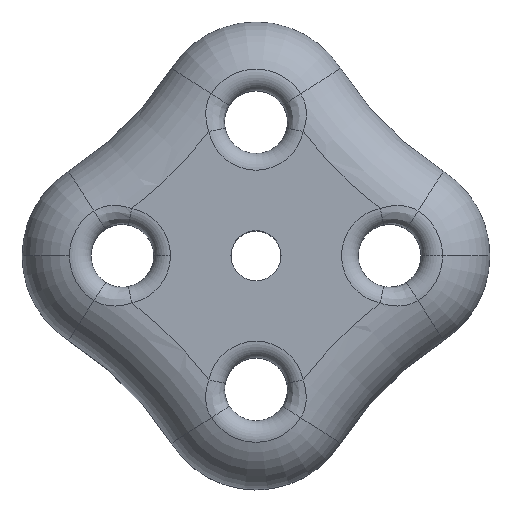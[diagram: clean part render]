
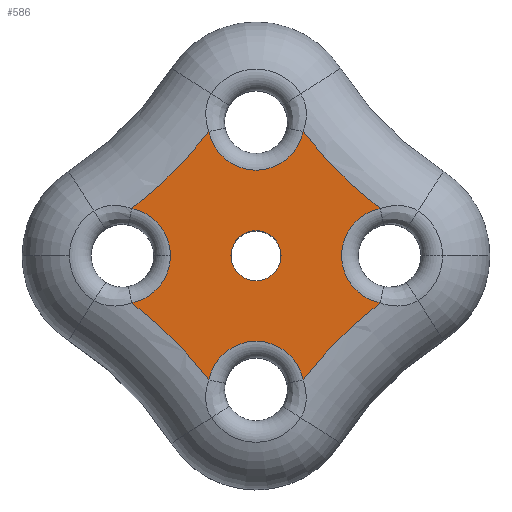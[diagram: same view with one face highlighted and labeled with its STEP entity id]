
A CAD part, top view. The second image highlights one B-rep face of the part: STEP entity #586.
In plain terms, the highlighted planar face has unit normal (0, 0, 1).
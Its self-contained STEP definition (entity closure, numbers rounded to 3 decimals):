
#58 = ORIENTED_EDGE ( 'NONE', *, *, #327, .T. ) ;
#70 = AXIS2_PLACEMENT_3D ( 'NONE', #1408, #176, #1596 ) ;
#99 = VERTEX_POINT ( 'NONE', #1064 ) ;
#125 = DIRECTION ( 'NONE',  ( 0., 0., -1. ) ) ;
#163 = DIRECTION ( 'NONE',  ( 0., 0., -1. ) ) ;
#176 = DIRECTION ( 'NONE',  ( 0., 0., -1. ) ) ;
#178 = ORIENTED_EDGE ( 'NONE', *, *, #2785, .T. ) ;
#207 = ORIENTED_EDGE ( 'NONE', *, *, #1687, .T. ) ;
#233 = ORIENTED_EDGE ( 'NONE', *, *, #2461, .T. ) ;
#250 = ORIENTED_EDGE ( 'NONE', *, *, #1040, .T. ) ;
#279 = DIRECTION ( 'NONE',  ( 0., 0., -1. ) ) ;
#296 = CARTESIAN_POINT ( 'NONE',  ( 18.596, -12.939, 40. ) ) ;
#327 = EDGE_CURVE ( 'NONE', #2051, #1508, #1218, .T. ) ;
#374 = EDGE_CURVE ( 'NONE', #944, #1015, #803, .T. ) ;
#385 = AXIS2_PLACEMENT_3D ( 'NONE', #996, #1192, #2840 ) ;
#425 = CARTESIAN_POINT ( 'NONE',  ( 0., 0., 40. ) ) ;
#512 = DIRECTION ( 'NONE',  ( 0., 0., -1. ) ) ;
#526 = DIRECTION ( 'NONE',  ( 0., 0., 1. ) ) ;
#549 = CARTESIAN_POINT ( 'NONE',  ( 0., -20., 40. ) ) ;
#586 = ADVANCED_FACE ( 'NONE', ( #755, #830 ), #2327, .T. ) ;
#620 = DIRECTION ( 'NONE',  ( 0., 0., -1. ) ) ;
#631 = DIRECTION ( 'NONE',  ( 1., 0., 0. ) ) ;
#655 = ORIENTED_EDGE ( 'NONE', *, *, #1025, .T. ) ;
#704 = ORIENTED_EDGE ( 'NONE', *, *, #374, .T. ) ;
#741 = ORIENTED_EDGE ( 'NONE', *, *, #2588, .T. ) ;
#749 = DIRECTION ( 'NONE',  ( 1., 0., 0. ) ) ;
#755 = FACE_BOUND ( 'NONE', #2675, .T. ) ;
#761 = DIRECTION ( 'NONE',  ( 0., 0., -1. ) ) ;
#803 = CIRCLE ( 'NONE', #902, 60. ) ;
#830 = FACE_OUTER_BOUND ( 'NONE', #2684, .T. ) ;
#902 = AXIS2_PLACEMENT_3D ( 'NONE', #1735, #512, #1986 ) ;
#917 = VERTEX_POINT ( 'NONE', #1810 ) ;
#941 = VERTEX_POINT ( 'NONE', #993 ) ;
#944 = VERTEX_POINT ( 'NONE', #2342 ) ;
#993 = CARTESIAN_POINT ( 'NONE',  ( -7.061, -1.404, 40. ) ) ;
#996 = CARTESIAN_POINT ( 'NONE',  ( 0., 0., 40. ) ) ;
#1015 = VERTEX_POINT ( 'NONE', #1845 ) ;
#1025 = EDGE_CURVE ( 'NONE', #2502, #944, #1178, .T. ) ;
#1040 = EDGE_CURVE ( 'NONE', #2185, #2502, #1114, .T. ) ;
#1064 = CARTESIAN_POINT ( 'NONE',  ( -3.75, -20., 40. ) ) ;
#1098 = VERTEX_POINT ( 'NONE', #2888 ) ;
#1114 = CIRCLE ( 'NONE', #2842, 7.199 ) ;
#1178 = CIRCLE ( 'NONE', #2854, 7.199 ) ;
#1192 = DIRECTION ( 'NONE',  ( 0., 0., 1. ) ) ;
#1218 = CIRCLE ( 'NONE', #70, 7.199 ) ;
#1224 = CARTESIAN_POINT ( 'NONE',  ( -20., -20., 40. ) ) ;
#1317 = CARTESIAN_POINT ( 'NONE',  ( -12.801, -20., 40. ) ) ;
#1355 = CARTESIAN_POINT ( 'NONE',  ( 0., -40., 40. ) ) ;
#1373 = CARTESIAN_POINT ( 'NONE',  ( -18.596, -12.939, 40. ) ) ;
#1383 = ORIENTED_EDGE ( 'NONE', *, *, #1917, .T. ) ;
#1387 = CARTESIAN_POINT ( 'NONE',  ( 54.861, -74.861, 40. ) ) ;
#1408 = CARTESIAN_POINT ( 'NONE',  ( 20., -20., 40. ) ) ;
#1420 = DIRECTION ( 'NONE',  ( 1., 0., 0. ) ) ;
#1506 = CARTESIAN_POINT ( 'NONE',  ( -54.861, 34.861, 40. ) ) ;
#1508 = VERTEX_POINT ( 'NONE', #296 ) ;
#1552 = DIRECTION ( 'NONE',  ( 1., 0., 0. ) ) ;
#1585 = DIRECTION ( 'NONE',  ( 1., 0., 0. ) ) ;
#1596 = DIRECTION ( 'NONE',  ( 1., 0., 0. ) ) ;
#1687 = EDGE_CURVE ( 'NONE', #1098, #941, #2693, .T. ) ;
#1721 = DIRECTION ( 'NONE',  ( 1., 0., 0. ) ) ;
#1735 = CARTESIAN_POINT ( 'NONE',  ( -54.861, -74.861, 40. ) ) ;
#1758 = CARTESIAN_POINT ( 'NONE',  ( 0., -20., 40. ) ) ;
#1810 = CARTESIAN_POINT ( 'NONE',  ( 7.061, -38.596, 40. ) ) ;
#1845 = CARTESIAN_POINT ( 'NONE',  ( -7.061, -38.596, 40. ) ) ;
#1853 = CARTESIAN_POINT ( 'NONE',  ( -20., -20., 40. ) ) ;
#1872 = DIRECTION ( 'NONE',  ( 0., 0., -1. ) ) ;
#1903 = CIRCLE ( 'NONE', #1969, 60. ) ;
#1917 = EDGE_CURVE ( 'NONE', #917, #2051, #2515, .T. ) ;
#1969 = AXIS2_PLACEMENT_3D ( 'NONE', #2043, #761, #2302 ) ;
#1986 = DIRECTION ( 'NONE',  ( 1., 0., 0. ) ) ;
#2005 = DIRECTION ( 'NONE',  ( 1., 0., 0. ) ) ;
#2017 = CARTESIAN_POINT ( 'NONE',  ( 3.75, -20., 40. ) ) ;
#2032 = DIRECTION ( 'NONE',  ( 0., 0., 1. ) ) ;
#2033 = CIRCLE ( 'NONE', #2075, 7.199 ) ;
#2036 = CIRCLE ( 'NONE', #2041, 3.75 ) ;
#2041 = AXIS2_PLACEMENT_3D ( 'NONE', #549, #2032, #749 ) ;
#2043 = CARTESIAN_POINT ( 'NONE',  ( 54.861, 34.861, 40. ) ) ;
#2051 = VERTEX_POINT ( 'NONE', #2488 ) ;
#2075 = AXIS2_PLACEMENT_3D ( 'NONE', #1355, #125, #1552 ) ;
#2081 = AXIS2_PLACEMENT_3D ( 'NONE', #1758, #526, #2005 ) ;
#2092 = CIRCLE ( 'NONE', #2081, 3.75 ) ;
#2115 = DIRECTION ( 'NONE',  ( 1., 0., 0. ) ) ;
#2136 = AXIS2_PLACEMENT_3D ( 'NONE', #1506, #279, #1721 ) ;
#2157 = CIRCLE ( 'NONE', #2136, 60. ) ;
#2185 = VERTEX_POINT ( 'NONE', #1373 ) ;
#2302 = DIRECTION ( 'NONE',  ( 1., 0., 0. ) ) ;
#2327 = PLANE ( 'NONE',  #385 ) ;
#2342 = CARTESIAN_POINT ( 'NONE',  ( -18.596, -27.061, 40. ) ) ;
#2419 = AXIS2_PLACEMENT_3D ( 'NONE', #1387, #163, #1585 ) ;
#2461 = EDGE_CURVE ( 'NONE', #941, #2185, #2157, .T. ) ;
#2488 = CARTESIAN_POINT ( 'NONE',  ( 18.596, -27.061, 40. ) ) ;
#2502 = VERTEX_POINT ( 'NONE', #1317 ) ;
#2515 = CIRCLE ( 'NONE', #2419, 60. ) ;
#2525 = AXIS2_PLACEMENT_3D ( 'NONE', #425, #1872, #631 ) ;
#2546 = EDGE_CURVE ( 'NONE', #2586, #99, #2092, .T. ) ;
#2586 = VERTEX_POINT ( 'NONE', #2017 ) ;
#2588 = EDGE_CURVE ( 'NONE', #1015, #917, #2033, .T. ) ;
#2589 = EDGE_CURVE ( 'NONE', #99, #2586, #2036, .T. ) ;
#2601 = ORIENTED_EDGE ( 'NONE', *, *, #2546, .F. ) ;
#2605 = ORIENTED_EDGE ( 'NONE', *, *, #2589, .F. ) ;
#2675 = EDGE_LOOP ( 'NONE', ( #2601, #2605 ) ) ;
#2684 = EDGE_LOOP ( 'NONE', ( #1383, #58, #178, #207, #233, #250, #655, #704, #741 ) ) ;
#2693 = CIRCLE ( 'NONE', #2525, 7.199 ) ;
#2785 = EDGE_CURVE ( 'NONE', #1508, #1098, #1903, .T. ) ;
#2840 = DIRECTION ( 'NONE',  ( 1., 0., 0. ) ) ;
#2842 = AXIS2_PLACEMENT_3D ( 'NONE', #1853, #620, #2115 ) ;
#2854 = AXIS2_PLACEMENT_3D ( 'NONE', #1224, #2869, #1420 ) ;
#2869 = DIRECTION ( 'NONE',  ( 0., 0., -1. ) ) ;
#2888 = CARTESIAN_POINT ( 'NONE',  ( 7.061, -1.404, 40. ) ) ;
